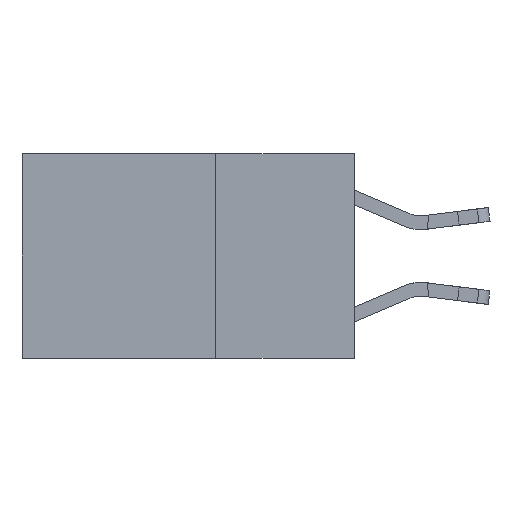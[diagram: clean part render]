
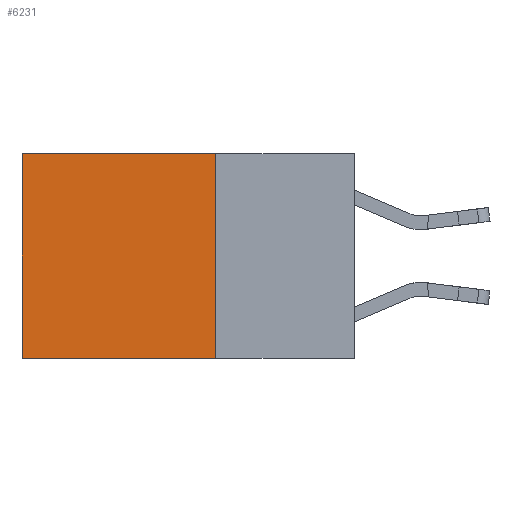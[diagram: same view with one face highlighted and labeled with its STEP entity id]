
A CAD part, left-side view. The second image highlights one B-rep face of the part: STEP entity #6231.
In plain terms, the highlighted planar face has unit normal (-1, 0, 0).
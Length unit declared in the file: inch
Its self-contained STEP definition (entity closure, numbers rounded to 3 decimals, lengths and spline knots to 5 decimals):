
#71 = EDGE_CURVE ( 'NONE', #11658, #3250, #12800, .T. ) ;
#144 = CARTESIAN_POINT ( 'NONE',  ( 0.2625, 0.25, 0. ) ) ;
#442 = CARTESIAN_POINT ( 'NONE',  ( 0.2625, 0.25, 0. ) ) ;
#757 = CARTESIAN_POINT ( 'NONE',  ( 0.2625, 0.25, 0. ) ) ;
#2843 = LINE ( 'NONE', #442, #13339 ) ;
#2924 = ORIENTED_EDGE ( 'NONE', *, *, #3974, .T. ) ;
#3250 = VERTEX_POINT ( 'NONE', #5487 ) ;
#3557 = CARTESIAN_POINT ( 'NONE',  ( 0.2625, 0.25, 0. ) ) ;
#3974 = EDGE_CURVE ( 'NONE', #12182, #3250, #4847, .T. ) ;
#4523 = ORIENTED_EDGE ( 'NONE', *, *, #8410, .F. ) ;
#4785 = DIRECTION ( 'NONE',  ( 0., 0., -1. ) ) ;
#4847 = LINE ( 'NONE', #6839, #7276 ) ;
#5487 = CARTESIAN_POINT ( 'NONE',  ( 0.2625, 0.6, -0.37 ) ) ;
#5549 = CARTESIAN_POINT ( 'NONE',  ( 0.2625, 0.6, 0. ) ) ;
#5659 = DIRECTION ( 'NONE',  ( 1., 0., 0. ) ) ;
#6231 = ADVANCED_FACE ( 'NONE', ( #9238 ), #12936, .F. ) ;
#6789 = VERTEX_POINT ( 'NONE', #144 ) ;
#6794 = ORIENTED_EDGE ( 'NONE', *, *, #13592, .T. ) ;
#6839 = CARTESIAN_POINT ( 'NONE',  ( 0.2625, 0.6, 0. ) ) ;
#6887 = DIRECTION ( 'NONE',  ( 0., 1., 0. ) ) ;
#7080 = CARTESIAN_POINT ( 'NONE',  ( 0.2625, 0.25, -0.37 ) ) ;
#7224 = VECTOR ( 'NONE', #7627, 39.37008 ) ;
#7276 = VECTOR ( 'NONE', #4785, 39.37008 ) ;
#7627 = DIRECTION ( 'NONE',  ( 0., 1., 0. ) ) ;
#8261 = DIRECTION ( 'NONE',  ( 0., 0., -1. ) ) ;
#8326 = ORIENTED_EDGE ( 'NONE', *, *, #71, .F. ) ;
#8410 = EDGE_CURVE ( 'NONE', #6789, #11658, #10382, .T. ) ;
#8944 = EDGE_LOOP ( 'NONE', ( #2924, #8326, #4523, #6794 ) ) ;
#9238 = FACE_OUTER_BOUND ( 'NONE', #8944, .T. ) ;
#9831 = AXIS2_PLACEMENT_3D ( 'NONE', #3557, #5659, #12975 ) ;
#10382 = LINE ( 'NONE', #757, #13121 ) ;
#11172 = CARTESIAN_POINT ( 'NONE',  ( 0.2625, 0.25, -0.37 ) ) ;
#11658 = VERTEX_POINT ( 'NONE', #11172 ) ;
#12182 = VERTEX_POINT ( 'NONE', #5549 ) ;
#12800 = LINE ( 'NONE', #7080, #7224 ) ;
#12936 = PLANE ( 'NONE',  #9831 ) ;
#12975 = DIRECTION ( 'NONE',  ( 0., 0., -1. ) ) ;
#13121 = VECTOR ( 'NONE', #8261, 39.37008 ) ;
#13339 = VECTOR ( 'NONE', #6887, 39.37008 ) ;
#13592 = EDGE_CURVE ( 'NONE', #6789, #12182, #2843, .T. ) ;
